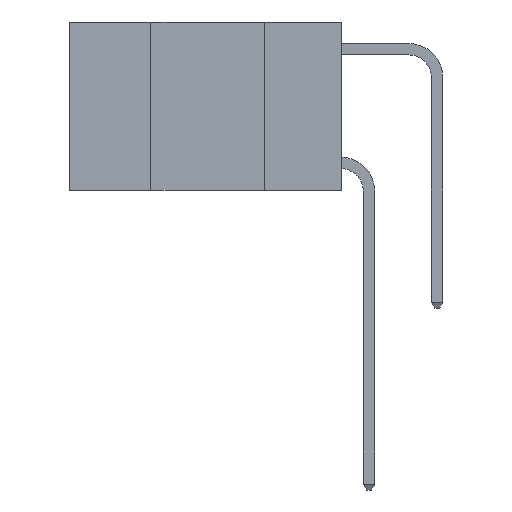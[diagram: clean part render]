
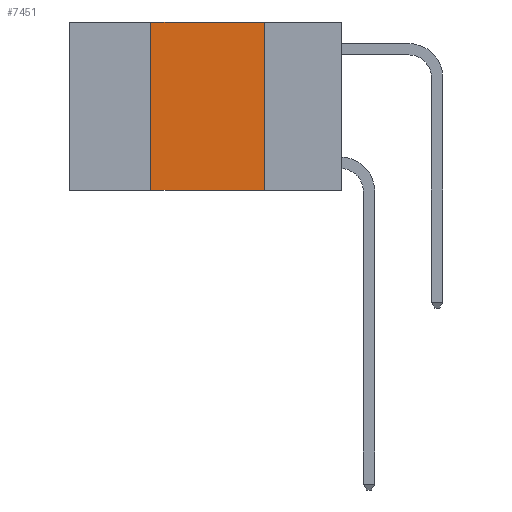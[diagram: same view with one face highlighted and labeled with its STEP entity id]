
A CAD part, left-side view. The second image highlights one B-rep face of the part: STEP entity #7451.
In plain terms, the highlighted planar face has unit normal (-1, 0, 0).
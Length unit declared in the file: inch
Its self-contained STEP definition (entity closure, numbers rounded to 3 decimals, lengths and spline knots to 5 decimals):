
#1005 = CARTESIAN_POINT ( 'NONE',  ( 0., 0.17, -0.37 ) ) ;
#1327 = FACE_OUTER_BOUND ( 'NONE', #3259, .T. ) ;
#1395 = VECTOR ( 'NONE', #6157, 39.37008 ) ;
#1847 = VERTEX_POINT ( 'NONE', #9595 ) ;
#2283 = CARTESIAN_POINT ( 'NONE',  ( 0., 0.6, -0.37 ) ) ;
#2521 = VERTEX_POINT ( 'NONE', #7152 ) ;
#2674 = DIRECTION ( 'NONE',  ( 0., 0., -1. ) ) ;
#2881 = CARTESIAN_POINT ( 'NONE',  ( 0., 0.17, 0. ) ) ;
#3207 = LINE ( 'NONE', #4363, #10783 ) ;
#3259 = EDGE_LOOP ( 'NONE', ( #7999, #8054, #7180, #6680 ) ) ;
#3389 = VERTEX_POINT ( 'NONE', #1005 ) ;
#3618 = CARTESIAN_POINT ( 'NONE',  ( 0., 0.6, 0. ) ) ;
#4043 = LINE ( 'NONE', #4622, #4379 ) ;
#4363 = CARTESIAN_POINT ( 'NONE',  ( 0., 0.42, 0. ) ) ;
#4379 = VECTOR ( 'NONE', #11183, 39.37008 ) ;
#4416 = EDGE_CURVE ( 'NONE', #10939, #2521, #4043, .T. ) ;
#4622 = CARTESIAN_POINT ( 'NONE',  ( 0., 0.6, 0. ) ) ;
#5360 = EDGE_CURVE ( 'NONE', #1847, #3389, #8821, .T. ) ;
#5547 = LINE ( 'NONE', #2881, #7778 ) ;
#5786 = DIRECTION ( 'NONE',  ( 0., 0., -1. ) ) ;
#6157 = DIRECTION ( 'NONE',  ( 0., -1., 0. ) ) ;
#6680 = ORIENTED_EDGE ( 'NONE', *, *, #5360, .T. ) ;
#7152 = CARTESIAN_POINT ( 'NONE',  ( 0., 0.17, 0. ) ) ;
#7180 = ORIENTED_EDGE ( 'NONE', *, *, #7285, .F. ) ;
#7285 = EDGE_CURVE ( 'NONE', #1847, #10939, #3207, .T. ) ;
#7451 = ADVANCED_FACE ( 'NONE', ( #1327 ), #12103, .F. ) ;
#7778 = VECTOR ( 'NONE', #5786, 39.37008 ) ;
#7999 = ORIENTED_EDGE ( 'NONE', *, *, #12046, .F. ) ;
#8054 = ORIENTED_EDGE ( 'NONE', *, *, #4416, .F. ) ;
#8444 = DIRECTION ( 'NONE',  ( 1., 0., 0. ) ) ;
#8821 = LINE ( 'NONE', #2283, #1395 ) ;
#9145 = CARTESIAN_POINT ( 'NONE',  ( 0., 0.42, 0. ) ) ;
#9595 = CARTESIAN_POINT ( 'NONE',  ( 0., 0.42, -0.37 ) ) ;
#9926 = AXIS2_PLACEMENT_3D ( 'NONE', #3618, #8444, #2674 ) ;
#10783 = VECTOR ( 'NONE', #11872, 39.37008 ) ;
#10939 = VERTEX_POINT ( 'NONE', #9145 ) ;
#11183 = DIRECTION ( 'NONE',  ( 0., -1., 0. ) ) ;
#11872 = DIRECTION ( 'NONE',  ( 0., 0., 1. ) ) ;
#12046 = EDGE_CURVE ( 'NONE', #2521, #3389, #5547, .T. ) ;
#12103 = PLANE ( 'NONE',  #9926 ) ;
